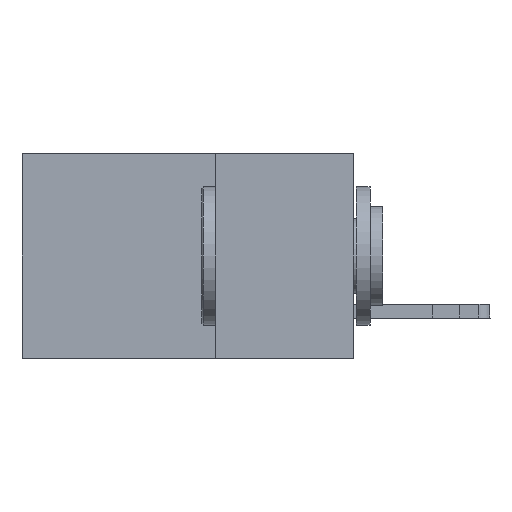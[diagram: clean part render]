
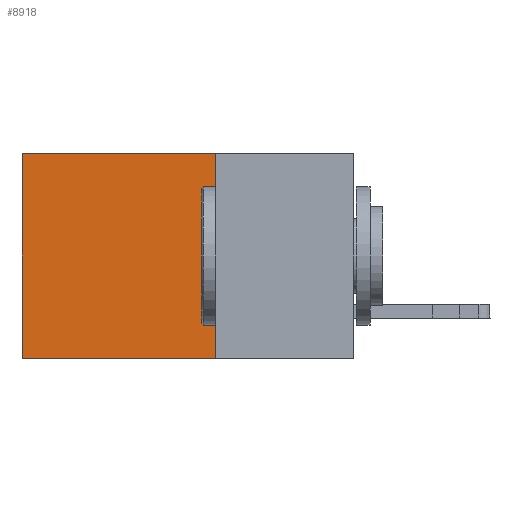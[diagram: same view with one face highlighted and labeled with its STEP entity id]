
A CAD part, left-side view. The second image highlights one B-rep face of the part: STEP entity #8918.
In plain terms, the highlighted planar face has unit normal (-1, 0, 0).
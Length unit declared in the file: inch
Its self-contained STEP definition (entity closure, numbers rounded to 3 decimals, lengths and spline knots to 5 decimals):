
#216 = VECTOR ( 'NONE', #14697, 39.37008 ) ;
#890 = LINE ( 'NONE', #12275, #17173 ) ;
#2694 = LINE ( 'NONE', #2820, #14834 ) ;
#2820 = CARTESIAN_POINT ( 'NONE',  ( 0.2875, 0.25, 0. ) ) ;
#2901 = CARTESIAN_POINT ( 'NONE',  ( 0.2875, 0.25, 0. ) ) ;
#4324 = VERTEX_POINT ( 'NONE', #2901 ) ;
#4538 = ORIENTED_EDGE ( 'NONE', *, *, #10404, .T. ) ;
#5086 = LINE ( 'NONE', #7106, #8822 ) ;
#6163 = CARTESIAN_POINT ( 'NONE',  ( 0.2875, 0.6, 0. ) ) ;
#6249 = VERTEX_POINT ( 'NONE', #6163 ) ;
#6545 = EDGE_CURVE ( 'NONE', #7792, #20255, #5086, .T. ) ;
#6916 = LINE ( 'NONE', #8308, #216 ) ;
#7106 = CARTESIAN_POINT ( 'NONE',  ( 0.2875, 0.25, -0.37 ) ) ;
#7792 = VERTEX_POINT ( 'NONE', #19760 ) ;
#7938 = DIRECTION ( 'NONE',  ( 0., 0., -1. ) ) ;
#8250 = EDGE_LOOP ( 'NONE', ( #14910, #16801, #17419, #4538 ) ) ;
#8308 = CARTESIAN_POINT ( 'NONE',  ( 0.2875, 0.6, 0. ) ) ;
#8822 = VECTOR ( 'NONE', #18686, 39.37008 ) ;
#8918 = ADVANCED_FACE ( 'NONE', ( #10903 ), #12818, .F. ) ;
#10404 = EDGE_CURVE ( 'NONE', #4324, #6249, #2694, .T. ) ;
#10903 = FACE_OUTER_BOUND ( 'NONE', #8250, .T. ) ;
#11126 = CARTESIAN_POINT ( 'NONE',  ( 0.2875, 0.25, 0. ) ) ;
#12275 = CARTESIAN_POINT ( 'NONE',  ( 0.2875, 0.25, 0. ) ) ;
#12605 = EDGE_CURVE ( 'NONE', #6249, #20255, #6916, .T. ) ;
#12818 = PLANE ( 'NONE',  #19959 ) ;
#14055 = DIRECTION ( 'NONE',  ( 0., 1., 0. ) ) ;
#14410 = DIRECTION ( 'NONE',  ( 1., 0., 0. ) ) ;
#14697 = DIRECTION ( 'NONE',  ( 0., 0., -1. ) ) ;
#14750 = EDGE_CURVE ( 'NONE', #4324, #7792, #890, .T. ) ;
#14834 = VECTOR ( 'NONE', #14055, 39.37008 ) ;
#14910 = ORIENTED_EDGE ( 'NONE', *, *, #12605, .T. ) ;
#16801 = ORIENTED_EDGE ( 'NONE', *, *, #6545, .F. ) ;
#17173 = VECTOR ( 'NONE', #7938, 39.37008 ) ;
#17419 = ORIENTED_EDGE ( 'NONE', *, *, #14750, .F. ) ;
#17525 = DIRECTION ( 'NONE',  ( 0., 0., -1. ) ) ;
#18686 = DIRECTION ( 'NONE',  ( 0., 1., 0. ) ) ;
#19651 = CARTESIAN_POINT ( 'NONE',  ( 0.2875, 0.6, -0.37 ) ) ;
#19760 = CARTESIAN_POINT ( 'NONE',  ( 0.2875, 0.25, -0.37 ) ) ;
#19959 = AXIS2_PLACEMENT_3D ( 'NONE', #11126, #14410, #17525 ) ;
#20255 = VERTEX_POINT ( 'NONE', #19651 ) ;
